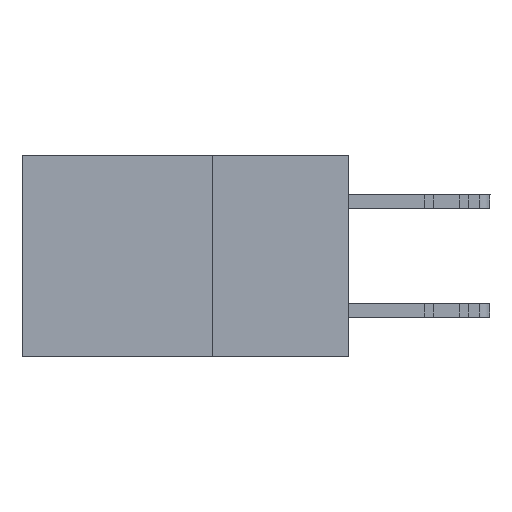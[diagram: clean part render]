
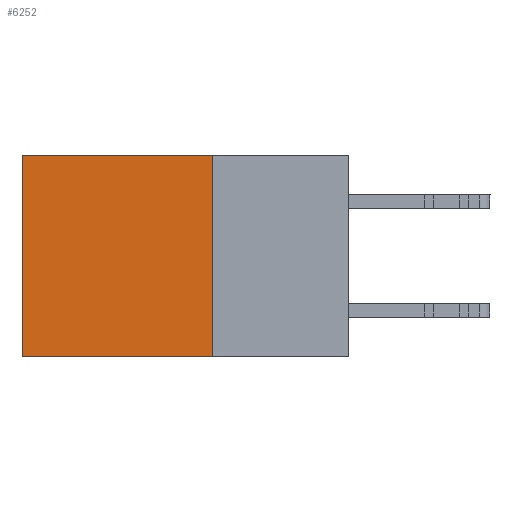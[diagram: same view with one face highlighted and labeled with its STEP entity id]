
A CAD part, left-side view. The second image highlights one B-rep face of the part: STEP entity #6252.
In plain terms, the highlighted planar face has unit normal (-1, 0, 0).
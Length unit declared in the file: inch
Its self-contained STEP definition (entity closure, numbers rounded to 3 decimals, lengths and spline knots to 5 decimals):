
#55 = LINE ( 'NONE', #19447, #19151 ) ;
#3228 = DIRECTION ( 'NONE',  ( 0., 1., 0. ) ) ;
#3521 = CARTESIAN_POINT ( 'NONE',  ( 0.298, 0.6, 0. ) ) ;
#5235 = ORIENTED_EDGE ( 'NONE', *, *, #29213, .F. ) ;
#5764 = DIRECTION ( 'NONE',  ( 0., 0., -1. ) ) ;
#6252 = ADVANCED_FACE ( 'NONE', ( #14635 ), #27227, .F. ) ;
#7375 = CARTESIAN_POINT ( 'NONE',  ( 0.298, 0.25, 0. ) ) ;
#8123 = LINE ( 'NONE', #18362, #29838 ) ;
#8613 = VERTEX_POINT ( 'NONE', #26630 ) ;
#8891 = VECTOR ( 'NONE', #3228, 39.37008 ) ;
#9806 = CARTESIAN_POINT ( 'NONE',  ( 0.298, 0.25, -0.37 ) ) ;
#10192 = DIRECTION ( 'NONE',  ( 0., 0., -1. ) ) ;
#10484 = LINE ( 'NONE', #19805, #8891 ) ;
#11121 = CARTESIAN_POINT ( 'NONE',  ( 0.298, 0.25, 0. ) ) ;
#11423 = EDGE_CURVE ( 'NONE', #8613, #22896, #30523, .T. ) ;
#12202 = VERTEX_POINT ( 'NONE', #24505 ) ;
#13761 = ORIENTED_EDGE ( 'NONE', *, *, #11423, .T. ) ;
#14635 = FACE_OUTER_BOUND ( 'NONE', #26702, .T. ) ;
#16725 = AXIS2_PLACEMENT_3D ( 'NONE', #7375, #29599, #10192 ) ;
#17826 = EDGE_CURVE ( 'NONE', #22896, #12202, #8123, .T. ) ;
#18362 = CARTESIAN_POINT ( 'NONE',  ( 0.298, 0.6, 0. ) ) ;
#18382 = DIRECTION ( 'NONE',  ( 0., 1., 0. ) ) ;
#19151 = VECTOR ( 'NONE', #29209, 39.37008 ) ;
#19447 = CARTESIAN_POINT ( 'NONE',  ( 0.298, 0.25, 0. ) ) ;
#19674 = EDGE_CURVE ( 'NONE', #21846, #12202, #10484, .T. ) ;
#19805 = CARTESIAN_POINT ( 'NONE',  ( 0.298, 0.25, -0.37 ) ) ;
#21846 = VERTEX_POINT ( 'NONE', #9806 ) ;
#22896 = VERTEX_POINT ( 'NONE', #3521 ) ;
#24505 = CARTESIAN_POINT ( 'NONE',  ( 0.298, 0.6, -0.37 ) ) ;
#26283 = VECTOR ( 'NONE', #18382, 39.37008 ) ;
#26630 = CARTESIAN_POINT ( 'NONE',  ( 0.298, 0.25, 0. ) ) ;
#26702 = EDGE_LOOP ( 'NONE', ( #30694, #30470, #5235, #13761 ) ) ;
#27227 = PLANE ( 'NONE',  #16725 ) ;
#29209 = DIRECTION ( 'NONE',  ( 0., 0., -1. ) ) ;
#29213 = EDGE_CURVE ( 'NONE', #8613, #21846, #55, .T. ) ;
#29599 = DIRECTION ( 'NONE',  ( 1., 0., 0. ) ) ;
#29838 = VECTOR ( 'NONE', #5764, 39.37008 ) ;
#30470 = ORIENTED_EDGE ( 'NONE', *, *, #19674, .F. ) ;
#30523 = LINE ( 'NONE', #11121, #26283 ) ;
#30694 = ORIENTED_EDGE ( 'NONE', *, *, #17826, .T. ) ;
